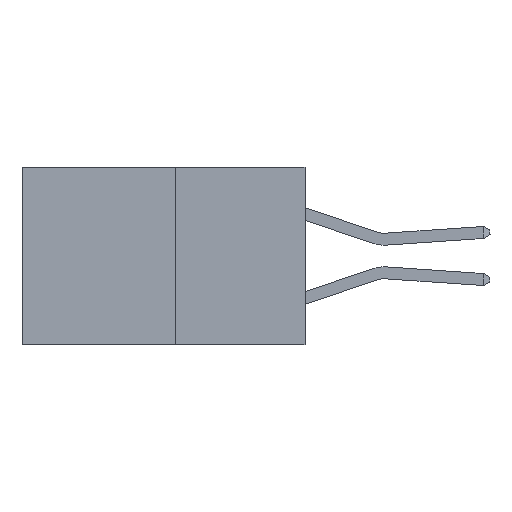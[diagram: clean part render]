
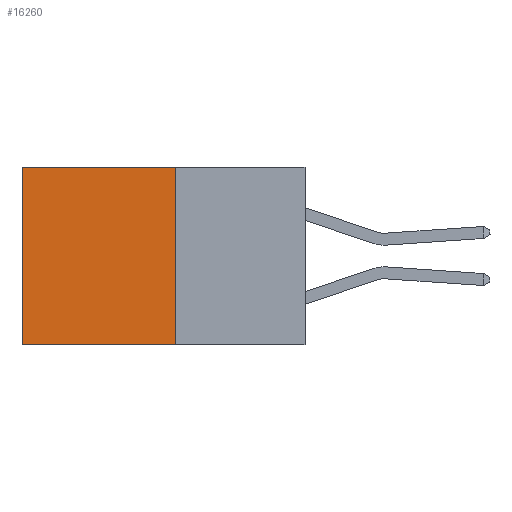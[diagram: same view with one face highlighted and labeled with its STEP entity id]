
A CAD part, left-side view. The second image highlights one B-rep face of the part: STEP entity #16260.
In plain terms, the highlighted planar face has unit normal (-1, 0, 0).
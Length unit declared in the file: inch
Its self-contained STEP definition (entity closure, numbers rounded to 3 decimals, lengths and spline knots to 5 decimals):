
#697 = ORIENTED_EDGE ( 'NONE', *, *, #9553, .F. ) ;
#1161 = DIRECTION ( 'NONE',  ( 0., 0., -1. ) ) ;
#1265 = DIRECTION ( 'NONE',  ( 0., 1., 0. ) ) ;
#2136 = EDGE_CURVE ( 'NONE', #23147, #3395, #17086, .T. ) ;
#3212 = CARTESIAN_POINT ( 'NONE',  ( 0.277, 0.27, -0.37 ) ) ;
#3395 = VERTEX_POINT ( 'NONE', #10064 ) ;
#3987 = ORIENTED_EDGE ( 'NONE', *, *, #4979, .T. ) ;
#4792 = VERTEX_POINT ( 'NONE', #23404 ) ;
#4979 = EDGE_CURVE ( 'NONE', #4792, #23147, #13470, .T. ) ;
#5759 = ORIENTED_EDGE ( 'NONE', *, *, #2136, .T. ) ;
#7457 = VERTEX_POINT ( 'NONE', #9823 ) ;
#8129 = VECTOR ( 'NONE', #14533, 39.37008 ) ;
#8506 = LINE ( 'NONE', #3212, #18595 ) ;
#9553 = EDGE_CURVE ( 'NONE', #4792, #7457, #8506, .T. ) ;
#9823 = CARTESIAN_POINT ( 'NONE',  ( 0.277, 0.27, -0.37 ) ) ;
#10064 = CARTESIAN_POINT ( 'NONE',  ( 0.277, 0.59, -0.37 ) ) ;
#10142 = ORIENTED_EDGE ( 'NONE', *, *, #17889, .F. ) ;
#11173 = PLANE ( 'NONE',  #17766 ) ;
#12570 = CARTESIAN_POINT ( 'NONE',  ( 0.277, 0.59, -0.37 ) ) ;
#13208 = DIRECTION ( 'NONE',  ( 0., 0., -1. ) ) ;
#13470 = LINE ( 'NONE', #14446, #8129 ) ;
#14446 = CARTESIAN_POINT ( 'NONE',  ( 0.277, 0.27, 0. ) ) ;
#14533 = DIRECTION ( 'NONE',  ( 0., 1., 0. ) ) ;
#16260 = ADVANCED_FACE ( 'NONE', ( #20745 ), #11173, .F. ) ;
#17086 = LINE ( 'NONE', #12570, #21091 ) ;
#17376 = CARTESIAN_POINT ( 'NONE',  ( 0.277, 0.27, -0.37 ) ) ;
#17766 = AXIS2_PLACEMENT_3D ( 'NONE', #23138, #25103, #13208 ) ;
#17889 = EDGE_CURVE ( 'NONE', #7457, #3395, #20347, .T. ) ;
#18595 = VECTOR ( 'NONE', #1161, 39.37008 ) ;
#19734 = VECTOR ( 'NONE', #1265, 39.37008 ) ;
#20347 = LINE ( 'NONE', #17376, #19734 ) ;
#20745 = FACE_OUTER_BOUND ( 'NONE', #20921, .T. ) ;
#20921 = EDGE_LOOP ( 'NONE', ( #5759, #10142, #697, #3987 ) ) ;
#21091 = VECTOR ( 'NONE', #25924, 39.37008 ) ;
#23138 = CARTESIAN_POINT ( 'NONE',  ( 0.277, 0.27, -0.37 ) ) ;
#23147 = VERTEX_POINT ( 'NONE', #24295 ) ;
#23404 = CARTESIAN_POINT ( 'NONE',  ( 0.277, 0.27, 0. ) ) ;
#24295 = CARTESIAN_POINT ( 'NONE',  ( 0.277, 0.59, 0. ) ) ;
#25103 = DIRECTION ( 'NONE',  ( 1., 0., 0. ) ) ;
#25924 = DIRECTION ( 'NONE',  ( 0., 0., -1. ) ) ;
